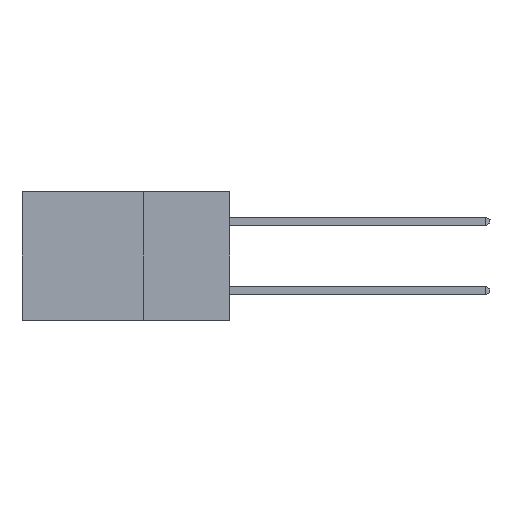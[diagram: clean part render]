
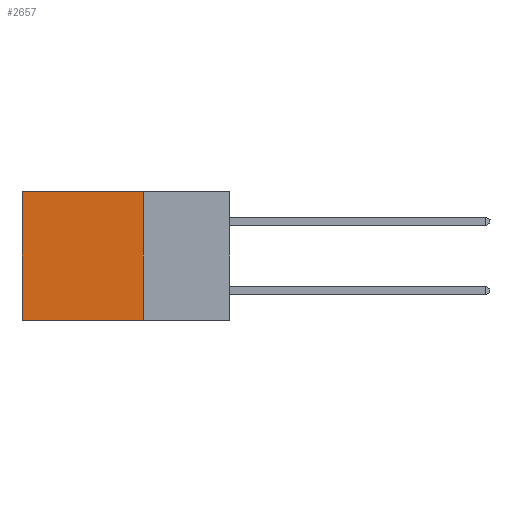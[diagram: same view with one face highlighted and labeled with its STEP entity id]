
A CAD part, left-side view. The second image highlights one B-rep face of the part: STEP entity #2657.
In plain terms, the highlighted planar face has unit normal (-1, 0, 0).
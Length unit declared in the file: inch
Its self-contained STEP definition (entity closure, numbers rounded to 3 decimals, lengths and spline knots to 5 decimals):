
#360 = LINE ( 'NONE', #16312, #13154 ) ;
#1713 = EDGE_CURVE ( 'NONE', #1917, #12839, #3608, .T. ) ;
#1917 = VERTEX_POINT ( 'NONE', #10963 ) ;
#2251 = ORIENTED_EDGE ( 'NONE', *, *, #1713, .F. ) ;
#2324 = VERTEX_POINT ( 'NONE', #3091 ) ;
#2657 = ADVANCED_FACE ( 'NONE', ( #13071 ), #10139, .F. ) ;
#3091 = CARTESIAN_POINT ( 'NONE',  ( 0.298, 0.6, 0. ) ) ;
#3608 = LINE ( 'NONE', #11125, #9574 ) ;
#4805 = EDGE_CURVE ( 'NONE', #15554, #2324, #360, .T. ) ;
#5088 = DIRECTION ( 'NONE',  ( 0., 0., -1. ) ) ;
#5473 = VECTOR ( 'NONE', #7887, 39.37008 ) ;
#6100 = EDGE_CURVE ( 'NONE', #15554, #1917, #14744, .T. ) ;
#6443 = CARTESIAN_POINT ( 'NONE',  ( 0.298, 0.25, 0. ) ) ;
#7602 = CARTESIAN_POINT ( 'NONE',  ( 0.298, 0.25, 0. ) ) ;
#7887 = DIRECTION ( 'NONE',  ( 0., 0., -1. ) ) ;
#8173 = DIRECTION ( 'NONE',  ( 0., 1., 0. ) ) ;
#8340 = CARTESIAN_POINT ( 'NONE',  ( 0.298, 0.6, -0.37 ) ) ;
#9574 = VECTOR ( 'NONE', #16804, 39.37008 ) ;
#10111 = EDGE_LOOP ( 'NONE', ( #11373, #2251, #16700, #13922 ) ) ;
#10139 = PLANE ( 'NONE',  #16749 ) ;
#10963 = CARTESIAN_POINT ( 'NONE',  ( 0.298, 0.25, -0.37 ) ) ;
#11125 = CARTESIAN_POINT ( 'NONE',  ( 0.298, 0.25, -0.37 ) ) ;
#11373 = ORIENTED_EDGE ( 'NONE', *, *, #14072, .T. ) ;
#12684 = VECTOR ( 'NONE', #15659, 39.37008 ) ;
#12839 = VERTEX_POINT ( 'NONE', #8340 ) ;
#13071 = FACE_OUTER_BOUND ( 'NONE', #10111, .T. ) ;
#13154 = VECTOR ( 'NONE', #8173, 39.37008 ) ;
#13172 = CARTESIAN_POINT ( 'NONE',  ( 0.298, 0.6, 0. ) ) ;
#13713 = LINE ( 'NONE', #13172, #5473 ) ;
#13922 = ORIENTED_EDGE ( 'NONE', *, *, #4805, .T. ) ;
#14072 = EDGE_CURVE ( 'NONE', #2324, #12839, #13713, .T. ) ;
#14744 = LINE ( 'NONE', #6443, #12684 ) ;
#15192 = CARTESIAN_POINT ( 'NONE',  ( 0.298, 0.25, 0. ) ) ;
#15554 = VERTEX_POINT ( 'NONE', #15192 ) ;
#15603 = DIRECTION ( 'NONE',  ( 1., 0., 0. ) ) ;
#15659 = DIRECTION ( 'NONE',  ( 0., 0., -1. ) ) ;
#16312 = CARTESIAN_POINT ( 'NONE',  ( 0.298, 0.25, 0. ) ) ;
#16700 = ORIENTED_EDGE ( 'NONE', *, *, #6100, .F. ) ;
#16749 = AXIS2_PLACEMENT_3D ( 'NONE', #7602, #15603, #5088 ) ;
#16804 = DIRECTION ( 'NONE',  ( 0., 1., 0. ) ) ;
